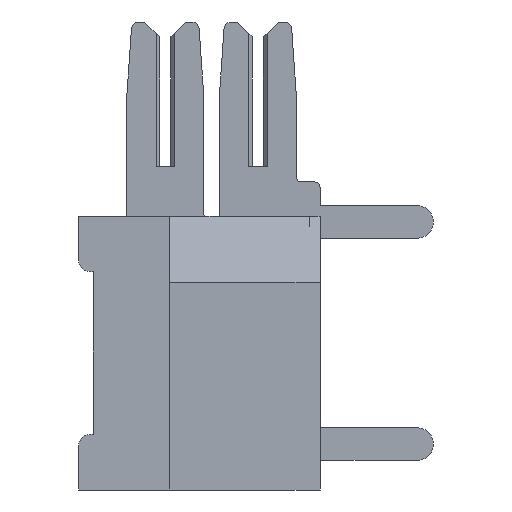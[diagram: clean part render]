
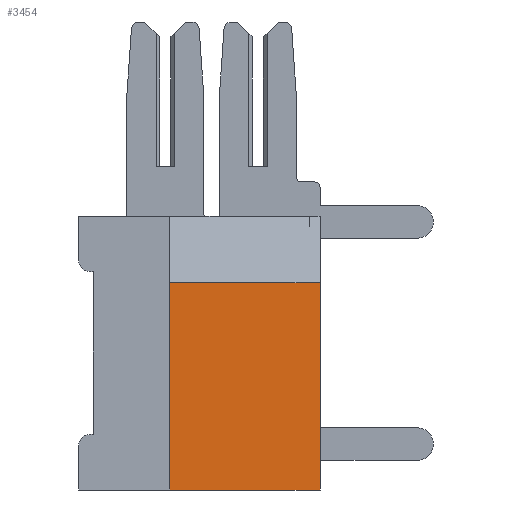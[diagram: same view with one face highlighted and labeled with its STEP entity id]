
A CAD part, left-side view. The second image highlights one B-rep face of the part: STEP entity #3454.
In plain terms, the highlighted planar face has unit normal (-1, 0, 0).
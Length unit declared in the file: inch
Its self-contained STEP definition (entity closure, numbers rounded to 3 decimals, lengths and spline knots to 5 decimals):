
#173 = LINE ( 'NONE', #2956, #1035 ) ;
#289 = CARTESIAN_POINT ( 'NONE',  ( 0., 0.203, -0.37 ) ) ;
#412 = LINE ( 'NONE', #1982, #5917 ) ;
#1009 = CARTESIAN_POINT ( 'NONE',  ( 0., 0.203, -0.37 ) ) ;
#1035 = VECTOR ( 'NONE', #10072, 39.37008 ) ;
#1143 = DIRECTION ( 'NONE',  ( 0., 0., -1. ) ) ;
#1831 = EDGE_CURVE ( 'NONE', #5059, #7923, #4533, .T. ) ;
#1921 = PLANE ( 'NONE',  #2973 ) ;
#1927 = DIRECTION ( 'NONE',  ( 0., 0., 1. ) ) ;
#1982 = CARTESIAN_POINT ( 'NONE',  ( 0., 0., 0. ) ) ;
#2074 = VERTEX_POINT ( 'NONE', #4473 ) ;
#2282 = CARTESIAN_POINT ( 'NONE',  ( 0., 0.326, -0.37 ) ) ;
#2804 = VERTEX_POINT ( 'NONE', #5882 ) ;
#2891 = DIRECTION ( 'NONE',  ( 1., 0., 0. ) ) ;
#2956 = CARTESIAN_POINT ( 'NONE',  ( 0., 0., -0.09 ) ) ;
#2973 = AXIS2_PLACEMENT_3D ( 'NONE', #5140, #2891, #1143 ) ;
#3132 = FACE_OUTER_BOUND ( 'NONE', #3198, .T. ) ;
#3198 = EDGE_LOOP ( 'NONE', ( #5622, #5885, #5077, #6632 ) ) ;
#3454 = ADVANCED_FACE ( 'NONE', ( #3132 ), #1921, .F. ) ;
#4473 = CARTESIAN_POINT ( 'NONE',  ( 0., 0., -0.09 ) ) ;
#4533 = LINE ( 'NONE', #1009, #5524 ) ;
#5059 = VERTEX_POINT ( 'NONE', #289 ) ;
#5077 = ORIENTED_EDGE ( 'NONE', *, *, #1831, .F. ) ;
#5140 = CARTESIAN_POINT ( 'NONE',  ( 0., 0.326, 0. ) ) ;
#5524 = VECTOR ( 'NONE', #1927, 39.37008 ) ;
#5622 = ORIENTED_EDGE ( 'NONE', *, *, #7177, .T. ) ;
#5882 = CARTESIAN_POINT ( 'NONE',  ( 0., 0., -0.37 ) ) ;
#5885 = ORIENTED_EDGE ( 'NONE', *, *, #6585, .T. ) ;
#5891 = LINE ( 'NONE', #2282, #7787 ) ;
#5917 = VECTOR ( 'NONE', #7618, 39.37008 ) ;
#6017 = CARTESIAN_POINT ( 'NONE',  ( 0., 0.203, -0.09 ) ) ;
#6585 = EDGE_CURVE ( 'NONE', #2074, #7923, #173, .T. ) ;
#6632 = ORIENTED_EDGE ( 'NONE', *, *, #8050, .T. ) ;
#7177 = EDGE_CURVE ( 'NONE', #2804, #2074, #412, .T. ) ;
#7618 = DIRECTION ( 'NONE',  ( 0., 0., 1. ) ) ;
#7787 = VECTOR ( 'NONE', #8631, 39.37008 ) ;
#7923 = VERTEX_POINT ( 'NONE', #6017 ) ;
#8050 = EDGE_CURVE ( 'NONE', #5059, #2804, #5891, .T. ) ;
#8631 = DIRECTION ( 'NONE',  ( 0., -1., 0. ) ) ;
#10072 = DIRECTION ( 'NONE',  ( 0., 1., 0. ) ) ;
